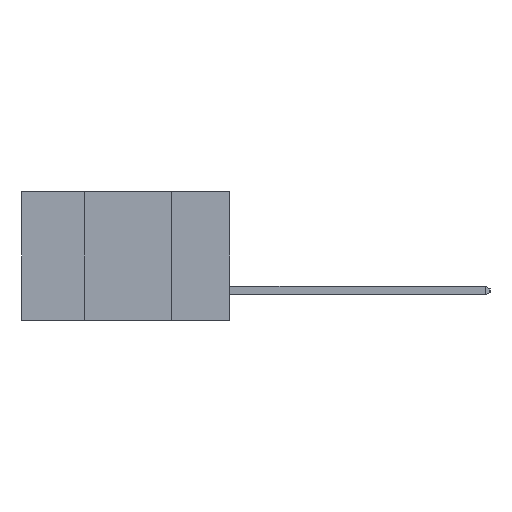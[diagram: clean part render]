
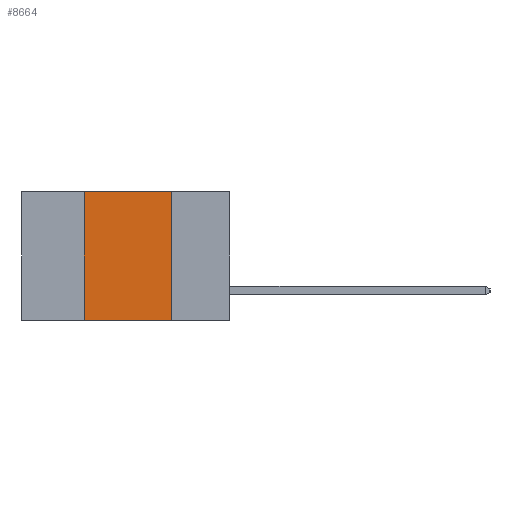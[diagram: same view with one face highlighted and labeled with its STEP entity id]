
A CAD part, left-side view. The second image highlights one B-rep face of the part: STEP entity #8664.
In plain terms, the highlighted planar face has unit normal (-1, 0, 0).
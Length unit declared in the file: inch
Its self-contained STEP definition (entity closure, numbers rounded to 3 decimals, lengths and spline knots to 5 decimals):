
#231 = VERTEX_POINT ( 'NONE', #5935 ) ;
#1169 = CARTESIAN_POINT ( 'NONE',  ( 0., 0.42, -0.37 ) ) ;
#2329 = ORIENTED_EDGE ( 'NONE', *, *, #14244, .F. ) ;
#2694 = VERTEX_POINT ( 'NONE', #10606 ) ;
#2918 = CARTESIAN_POINT ( 'NONE',  ( 0., 0.42, -0.37 ) ) ;
#2951 = VECTOR ( 'NONE', #11519, 39.37008 ) ;
#3876 = EDGE_CURVE ( 'NONE', #12001, #231, #7989, .T. ) ;
#4134 = DIRECTION ( 'NONE',  ( 0., 0., 1. ) ) ;
#4306 = VECTOR ( 'NONE', #4134, 39.37008 ) ;
#4406 = PLANE ( 'NONE',  #9750 ) ;
#4444 = EDGE_CURVE ( 'NONE', #6837, #231, #6132, .T. ) ;
#5853 = EDGE_LOOP ( 'NONE', ( #12645, #2329, #9903, #13851 ) ) ;
#5935 = CARTESIAN_POINT ( 'NONE',  ( 0., 0.17, -0.37 ) ) ;
#6132 = LINE ( 'NONE', #11568, #2951 ) ;
#6744 = DIRECTION ( 'NONE',  ( 0., 0., -1. ) ) ;
#6837 = VERTEX_POINT ( 'NONE', #1169 ) ;
#7083 = VECTOR ( 'NONE', #12041, 39.37008 ) ;
#7989 = LINE ( 'NONE', #14381, #8343 ) ;
#8039 = FACE_OUTER_BOUND ( 'NONE', #5853, .T. ) ;
#8343 = VECTOR ( 'NONE', #13847, 39.37008 ) ;
#8664 = ADVANCED_FACE ( 'NONE', ( #8039 ), #4406, .F. ) ;
#9159 = EDGE_CURVE ( 'NONE', #6837, #2694, #10851, .T. ) ;
#9739 = CARTESIAN_POINT ( 'NONE',  ( 0., 0.6, 0. ) ) ;
#9750 = AXIS2_PLACEMENT_3D ( 'NONE', #12513, #13683, #6744 ) ;
#9903 = ORIENTED_EDGE ( 'NONE', *, *, #9159, .F. ) ;
#10170 = LINE ( 'NONE', #9739, #7083 ) ;
#10606 = CARTESIAN_POINT ( 'NONE',  ( 0., 0.42, 0. ) ) ;
#10851 = LINE ( 'NONE', #2918, #4306 ) ;
#11519 = DIRECTION ( 'NONE',  ( 0., -1., 0. ) ) ;
#11568 = CARTESIAN_POINT ( 'NONE',  ( 0., 0.6, -0.37 ) ) ;
#11941 = CARTESIAN_POINT ( 'NONE',  ( 0., 0.17, 0. ) ) ;
#12001 = VERTEX_POINT ( 'NONE', #11941 ) ;
#12041 = DIRECTION ( 'NONE',  ( 0., -1., 0. ) ) ;
#12513 = CARTESIAN_POINT ( 'NONE',  ( 0., 0.6, 0. ) ) ;
#12645 = ORIENTED_EDGE ( 'NONE', *, *, #3876, .F. ) ;
#13683 = DIRECTION ( 'NONE',  ( 1., 0., 0. ) ) ;
#13847 = DIRECTION ( 'NONE',  ( 0., 0., -1. ) ) ;
#13851 = ORIENTED_EDGE ( 'NONE', *, *, #4444, .T. ) ;
#14244 = EDGE_CURVE ( 'NONE', #2694, #12001, #10170, .T. ) ;
#14381 = CARTESIAN_POINT ( 'NONE',  ( 0., 0.17, -0.37 ) ) ;
